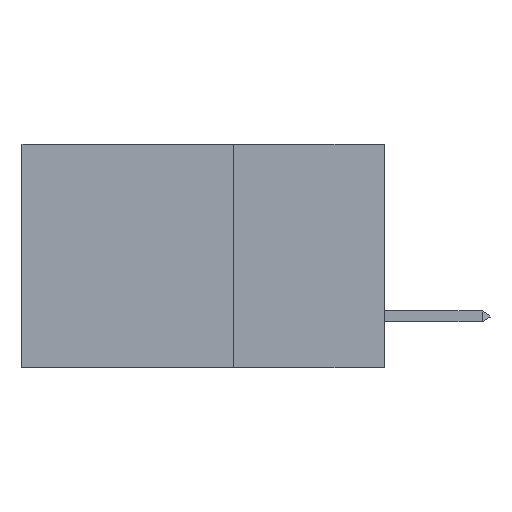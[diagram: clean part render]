
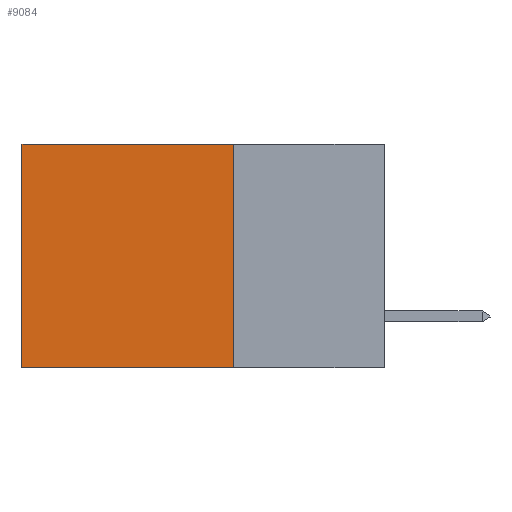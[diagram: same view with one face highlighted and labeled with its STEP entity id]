
A CAD part, left-side view. The second image highlights one B-rep face of the part: STEP entity #9084.
In plain terms, the highlighted planar face has unit normal (-1, 0, 0).
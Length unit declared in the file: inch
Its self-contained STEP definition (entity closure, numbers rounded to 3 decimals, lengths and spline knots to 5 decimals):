
#68 = ORIENTED_EDGE ( 'NONE', *, *, #19776, .T. ) ;
#187 = EDGE_CURVE ( 'NONE', #5898, #12977, #8531, .T. ) ;
#224 = AXIS2_PLACEMENT_3D ( 'NONE', #5847, #20846, #18943 ) ;
#565 = CARTESIAN_POINT ( 'NONE',  ( 0.2875, 0.6, 0. ) ) ;
#3156 = EDGE_CURVE ( 'NONE', #21155, #17570, #18604, .T. ) ;
#3387 = CARTESIAN_POINT ( 'NONE',  ( 0.2875, 0.25, 0. ) ) ;
#3513 = FACE_OUTER_BOUND ( 'NONE', #10207, .T. ) ;
#4186 = VECTOR ( 'NONE', #7031, 39.37008 ) ;
#5847 = CARTESIAN_POINT ( 'NONE',  ( 0.2875, 0.25, 0. ) ) ;
#5898 = VERTEX_POINT ( 'NONE', #12877 ) ;
#6294 = CARTESIAN_POINT ( 'NONE',  ( 0.2875, 0.25, -0.37 ) ) ;
#7031 = DIRECTION ( 'NONE',  ( 0., 0., -1. ) ) ;
#7161 = DIRECTION ( 'NONE',  ( 0., 0., -1. ) ) ;
#7585 = PLANE ( 'NONE',  #224 ) ;
#7698 = EDGE_CURVE ( 'NONE', #21155, #5898, #19135, .T. ) ;
#8531 = LINE ( 'NONE', #6294, #23181 ) ;
#9084 = ADVANCED_FACE ( 'NONE', ( #3513 ), #7585, .F. ) ;
#10207 = EDGE_LOOP ( 'NONE', ( #68, #15763, #12138, #21406 ) ) ;
#10796 = CARTESIAN_POINT ( 'NONE',  ( 0.2875, 0.25, 0. ) ) ;
#11939 = DIRECTION ( 'NONE',  ( 0., 1., 0. ) ) ;
#12138 = ORIENTED_EDGE ( 'NONE', *, *, #7698, .F. ) ;
#12252 = LINE ( 'NONE', #22078, #23406 ) ;
#12877 = CARTESIAN_POINT ( 'NONE',  ( 0.2875, 0.25, -0.37 ) ) ;
#12977 = VERTEX_POINT ( 'NONE', #13592 ) ;
#13592 = CARTESIAN_POINT ( 'NONE',  ( 0.2875, 0.6, -0.37 ) ) ;
#15763 = ORIENTED_EDGE ( 'NONE', *, *, #187, .F. ) ;
#16238 = DIRECTION ( 'NONE',  ( 0., 1., 0. ) ) ;
#17570 = VERTEX_POINT ( 'NONE', #565 ) ;
#18604 = LINE ( 'NONE', #3387, #18910 ) ;
#18910 = VECTOR ( 'NONE', #16238, 39.37008 ) ;
#18943 = DIRECTION ( 'NONE',  ( 0., 0., -1. ) ) ;
#19075 = CARTESIAN_POINT ( 'NONE',  ( 0.2875, 0.25, 0. ) ) ;
#19135 = LINE ( 'NONE', #10796, #4186 ) ;
#19776 = EDGE_CURVE ( 'NONE', #17570, #12977, #12252, .T. ) ;
#20846 = DIRECTION ( 'NONE',  ( 1., 0., 0. ) ) ;
#21155 = VERTEX_POINT ( 'NONE', #19075 ) ;
#21406 = ORIENTED_EDGE ( 'NONE', *, *, #3156, .T. ) ;
#22078 = CARTESIAN_POINT ( 'NONE',  ( 0.2875, 0.6, 0. ) ) ;
#23181 = VECTOR ( 'NONE', #11939, 39.37008 ) ;
#23406 = VECTOR ( 'NONE', #7161, 39.37008 ) ;
